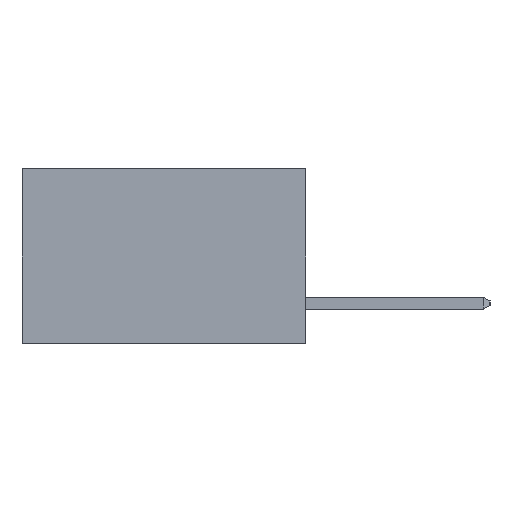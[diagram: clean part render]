
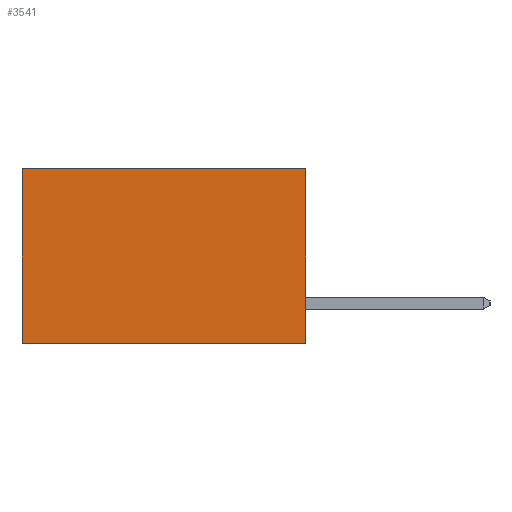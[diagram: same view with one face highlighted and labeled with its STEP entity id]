
A CAD part, left-side view. The second image highlights one B-rep face of the part: STEP entity #3541.
In plain terms, the highlighted planar face has unit normal (-1, 0, 0).
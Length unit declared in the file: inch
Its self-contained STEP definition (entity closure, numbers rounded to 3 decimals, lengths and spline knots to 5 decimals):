
#796 = LINE ( 'NONE', #10188, #7330 ) ;
#798 = ORIENTED_EDGE ( 'NONE', *, *, #1618, .F. ) ;
#1575 = EDGE_CURVE ( 'NONE', #10828, #7582, #8120, .T. ) ;
#1618 = EDGE_CURVE ( 'NONE', #8540, #10828, #796, .T. ) ;
#1741 = ORIENTED_EDGE ( 'NONE', *, *, #2198, .T. ) ;
#1811 = DIRECTION ( 'NONE',  ( 0., 0., -1. ) ) ;
#1838 = DIRECTION ( 'NONE',  ( 1., 0., 0. ) ) ;
#2198 = EDGE_CURVE ( 'NONE', #8540, #7151, #5052, .T. ) ;
#2206 = EDGE_LOOP ( 'NONE', ( #7263, #5253, #798, #1741 ) ) ;
#2836 = PLANE ( 'NONE',  #6878 ) ;
#3205 = CARTESIAN_POINT ( 'NONE',  ( 0.2615, 0.6, -0.37 ) ) ;
#3329 = CARTESIAN_POINT ( 'NONE',  ( 0.2615, 0., -0.37 ) ) ;
#3541 = ADVANCED_FACE ( 'NONE', ( #11184 ), #2836, .F. ) ;
#3930 = CARTESIAN_POINT ( 'NONE',  ( 0.2615, 0., 0. ) ) ;
#4685 = CARTESIAN_POINT ( 'NONE',  ( 0.2615, 0., -0.37 ) ) ;
#5052 = LINE ( 'NONE', #8709, #7033 ) ;
#5253 = ORIENTED_EDGE ( 'NONE', *, *, #1575, .F. ) ;
#5281 = CARTESIAN_POINT ( 'NONE',  ( 0.2615, 0., -0.37 ) ) ;
#5822 = EDGE_CURVE ( 'NONE', #7151, #7582, #6706, .T. ) ;
#6076 = CARTESIAN_POINT ( 'NONE',  ( 0.2615, 0.6, -0.37 ) ) ;
#6105 = VECTOR ( 'NONE', #11143, 39.37008 ) ;
#6432 = VECTOR ( 'NONE', #8393, 39.37008 ) ;
#6706 = LINE ( 'NONE', #3205, #6432 ) ;
#6878 = AXIS2_PLACEMENT_3D ( 'NONE', #3329, #1838, #1811 ) ;
#7033 = VECTOR ( 'NONE', #7390, 39.37008 ) ;
#7151 = VERTEX_POINT ( 'NONE', #11410 ) ;
#7263 = ORIENTED_EDGE ( 'NONE', *, *, #5822, .T. ) ;
#7330 = VECTOR ( 'NONE', #10326, 39.37008 ) ;
#7390 = DIRECTION ( 'NONE',  ( 0., 1., 0. ) ) ;
#7582 = VERTEX_POINT ( 'NONE', #6076 ) ;
#8120 = LINE ( 'NONE', #5281, #6105 ) ;
#8393 = DIRECTION ( 'NONE',  ( 0., 0., -1. ) ) ;
#8540 = VERTEX_POINT ( 'NONE', #3930 ) ;
#8709 = CARTESIAN_POINT ( 'NONE',  ( 0.2615, 0., 0. ) ) ;
#10188 = CARTESIAN_POINT ( 'NONE',  ( 0.2615, 0., -0.37 ) ) ;
#10326 = DIRECTION ( 'NONE',  ( 0., 0., -1. ) ) ;
#10828 = VERTEX_POINT ( 'NONE', #4685 ) ;
#11143 = DIRECTION ( 'NONE',  ( 0., 1., 0. ) ) ;
#11184 = FACE_OUTER_BOUND ( 'NONE', #2206, .T. ) ;
#11410 = CARTESIAN_POINT ( 'NONE',  ( 0.2615, 0.6, 0. ) ) ;
